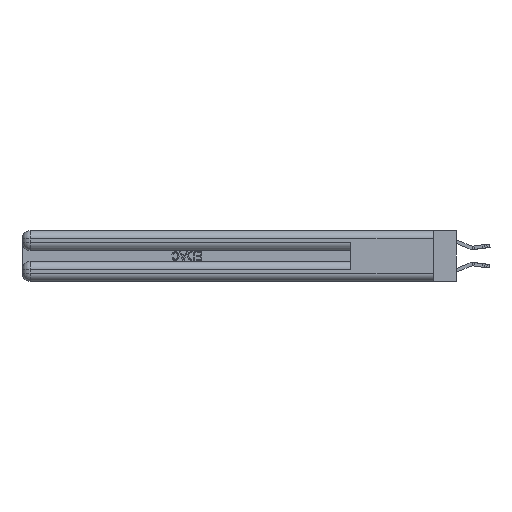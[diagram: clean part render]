
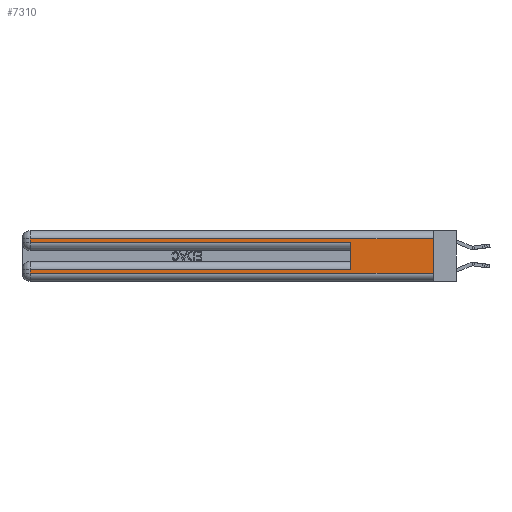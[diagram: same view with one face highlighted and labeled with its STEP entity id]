
A CAD part, left-side view. The second image highlights one B-rep face of the part: STEP entity #7310.
In plain terms, the highlighted planar face has unit normal (-1, 0, 0).
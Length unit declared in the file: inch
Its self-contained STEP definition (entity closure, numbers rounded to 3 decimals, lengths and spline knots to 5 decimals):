
#416 = VECTOR ( 'NONE', #17268, 39.37008 ) ;
#625 = VERTEX_POINT ( 'NONE', #25030 ) ;
#745 = VERTEX_POINT ( 'NONE', #22821 ) ;
#1063 = LINE ( 'NONE', #5934, #26292 ) ;
#2083 = EDGE_CURVE ( 'NONE', #18338, #20046, #14433, .T. ) ;
#4403 = DIRECTION ( 'NONE',  ( 0., 0., -1. ) ) ;
#5593 = LINE ( 'NONE', #12561, #9887 ) ;
#5908 = VECTOR ( 'NONE', #21676, 39.37008 ) ;
#5934 = CARTESIAN_POINT ( 'NONE',  ( 0., 0., 0.085 ) ) ;
#5952 = VERTEX_POINT ( 'NONE', #6616 ) ;
#6592 = LINE ( 'NONE', #30823, #26615 ) ;
#6616 = CARTESIAN_POINT ( 'NONE',  ( 0., 2.94, 0.085 ) ) ;
#7234 = CARTESIAN_POINT ( 'NONE',  ( 0., 2.94, 0.06 ) ) ;
#7310 = ADVANCED_FACE ( 'NONE', ( #13759 ), #23286, .F. ) ;
#7461 = CARTESIAN_POINT ( 'NONE',  ( 0., 0., 0.37 ) ) ;
#7610 = AXIS2_PLACEMENT_3D ( 'NONE', #25819, #10775, #28319 ) ;
#7990 = LINE ( 'NONE', #14748, #416 ) ;
#8260 = LINE ( 'NONE', #7461, #14925 ) ;
#8444 = ORIENTED_EDGE ( 'NONE', *, *, #20660, .T. ) ;
#8899 = EDGE_CURVE ( 'NONE', #5952, #18338, #15027, .T. ) ;
#9433 = CARTESIAN_POINT ( 'NONE',  ( 0., 0., 0.06 ) ) ;
#9887 = VECTOR ( 'NONE', #15083, 39.37008 ) ;
#9966 = DIRECTION ( 'NONE',  ( 0., 0., -1. ) ) ;
#10549 = DIRECTION ( 'NONE',  ( 0., -1., 0. ) ) ;
#10573 = EDGE_CURVE ( 'NONE', #32532, #5952, #1063, .T. ) ;
#10775 = DIRECTION ( 'NONE',  ( 1., 0., 0. ) ) ;
#10897 = DIRECTION ( 'NONE',  ( 0., 0., 1. ) ) ;
#11285 = ORIENTED_EDGE ( 'NONE', *, *, #12251, .F. ) ;
#12251 = EDGE_CURVE ( 'NONE', #32532, #32315, #6592, .T. ) ;
#12561 = CARTESIAN_POINT ( 'NONE',  ( 0., 0., 0.31 ) ) ;
#12863 = ORIENTED_EDGE ( 'NONE', *, *, #10573, .T. ) ;
#13602 = DIRECTION ( 'NONE',  ( 0., 1., 0. ) ) ;
#13759 = FACE_OUTER_BOUND ( 'NONE', #29243, .T. ) ;
#14433 = LINE ( 'NONE', #23060, #26989 ) ;
#14445 = ORIENTED_EDGE ( 'NONE', *, *, #2083, .T. ) ;
#14748 = CARTESIAN_POINT ( 'NONE',  ( 0., 0., 0.285 ) ) ;
#14925 = VECTOR ( 'NONE', #9966, 39.37008 ) ;
#15027 = LINE ( 'NONE', #31914, #27568 ) ;
#15083 = DIRECTION ( 'NONE',  ( 0., 1., 0. ) ) ;
#16379 = ORIENTED_EDGE ( 'NONE', *, *, #19009, .T. ) ;
#17162 = VERTEX_POINT ( 'NONE', #27860 ) ;
#17176 = CARTESIAN_POINT ( 'NONE',  ( 0., 0.6, 0.285 ) ) ;
#17268 = DIRECTION ( 'NONE',  ( 0., -1., 0. ) ) ;
#18338 = VERTEX_POINT ( 'NONE', #7234 ) ;
#19009 = EDGE_CURVE ( 'NONE', #17162, #32315, #7990, .T. ) ;
#19172 = CARTESIAN_POINT ( 'NONE',  ( 0., 2.94, 0.37 ) ) ;
#19265 = LINE ( 'NONE', #19172, #5908 ) ;
#20046 = VERTEX_POINT ( 'NONE', #9433 ) ;
#20467 = CARTESIAN_POINT ( 'NONE',  ( 0., 0.6, 0.085 ) ) ;
#20660 = EDGE_CURVE ( 'NONE', #745, #17162, #19265, .T. ) ;
#21676 = DIRECTION ( 'NONE',  ( 0., 0., -1. ) ) ;
#22237 = ORIENTED_EDGE ( 'NONE', *, *, #29051, .F. ) ;
#22345 = EDGE_CURVE ( 'NONE', #625, #745, #5593, .T. ) ;
#22821 = CARTESIAN_POINT ( 'NONE',  ( 0., 2.94, 0.31 ) ) ;
#23060 = CARTESIAN_POINT ( 'NONE',  ( 0., 0., 0.06 ) ) ;
#23286 = PLANE ( 'NONE',  #7610 ) ;
#25030 = CARTESIAN_POINT ( 'NONE',  ( 0., 0., 0.31 ) ) ;
#25819 = CARTESIAN_POINT ( 'NONE',  ( 0., 0., 0.37 ) ) ;
#26131 = ORIENTED_EDGE ( 'NONE', *, *, #22345, .T. ) ;
#26224 = ORIENTED_EDGE ( 'NONE', *, *, #8899, .T. ) ;
#26292 = VECTOR ( 'NONE', #13602, 39.37008 ) ;
#26615 = VECTOR ( 'NONE', #10897, 39.37008 ) ;
#26989 = VECTOR ( 'NONE', #10549, 39.37008 ) ;
#27568 = VECTOR ( 'NONE', #4403, 39.37008 ) ;
#27860 = CARTESIAN_POINT ( 'NONE',  ( 0., 2.94, 0.285 ) ) ;
#28319 = DIRECTION ( 'NONE',  ( 0., 0., -1. ) ) ;
#29051 = EDGE_CURVE ( 'NONE', #625, #20046, #8260, .T. ) ;
#29243 = EDGE_LOOP ( 'NONE', ( #22237, #26131, #8444, #16379, #11285, #12863, #26224, #14445 ) ) ;
#30823 = CARTESIAN_POINT ( 'NONE',  ( 0., 0.6, 0.145 ) ) ;
#31914 = CARTESIAN_POINT ( 'NONE',  ( 0., 2.94, 0.37 ) ) ;
#32315 = VERTEX_POINT ( 'NONE', #17176 ) ;
#32532 = VERTEX_POINT ( 'NONE', #20467 ) ;
